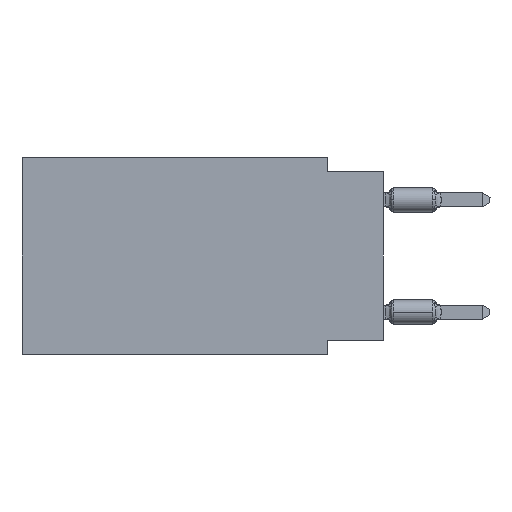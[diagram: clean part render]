
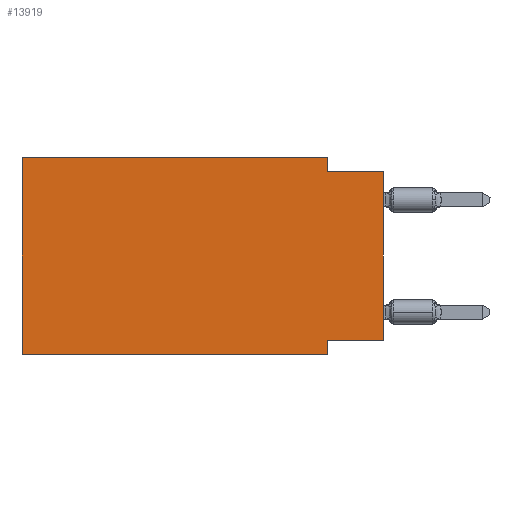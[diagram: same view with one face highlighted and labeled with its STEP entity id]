
A CAD part, left-side view. The second image highlights one B-rep face of the part: STEP entity #13919.
In plain terms, the highlighted planar face has unit normal (-1, 0, 0).
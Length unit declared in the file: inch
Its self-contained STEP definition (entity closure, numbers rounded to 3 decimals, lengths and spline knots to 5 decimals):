
#521 = EDGE_CURVE ( 'NONE', #18550, #58341, #49452, .T. ) ;
#3429 = CARTESIAN_POINT ( 'NONE',  ( 0., 0.1, 0. ) ) ;
#7042 = PLANE ( 'NONE',  #61898 ) ;
#7747 = FACE_OUTER_BOUND ( 'NONE', #23173, .T. ) ;
#7822 = CARTESIAN_POINT ( 'NONE',  ( 0., 0., 0. ) ) ;
#8742 = ORIENTED_EDGE ( 'NONE', *, *, #59085, .F. ) ;
#11381 = CARTESIAN_POINT ( 'NONE',  ( 0., 0.1, -0.025 ) ) ;
#11712 = CARTESIAN_POINT ( 'NONE',  ( 0., 0.1, -0.35 ) ) ;
#11769 = VERTEX_POINT ( 'NONE', #45825 ) ;
#12940 = VECTOR ( 'NONE', #59813, 39.37008 ) ;
#13713 = LINE ( 'NONE', #46192, #62408 ) ;
#13919 = ADVANCED_FACE ( 'NONE', ( #7747 ), #7042, .F. ) ;
#14880 = VERTEX_POINT ( 'NONE', #69265 ) ;
#18035 = LINE ( 'NONE', #50842, #18871 ) ;
#18550 = VERTEX_POINT ( 'NONE', #19063 ) ;
#18871 = VECTOR ( 'NONE', #55851, 39.37008 ) ;
#19063 = CARTESIAN_POINT ( 'NONE',  ( 0., 0.1, -0.325 ) ) ;
#20059 = VECTOR ( 'NONE', #61275, 39.37008 ) ;
#21647 = DIRECTION ( 'NONE',  ( 0., 1., 0. ) ) ;
#23173 = EDGE_LOOP ( 'NONE', ( #65685, #52753, #58268, #8742, #44188, #50461, #50908, #44520 ) ) ;
#24486 = DIRECTION ( 'NONE',  ( 1., 0., 0. ) ) ;
#24844 = DIRECTION ( 'NONE',  ( 0., -1., 0. ) ) ;
#25246 = EDGE_CURVE ( 'NONE', #11769, #18550, #44127, .T. ) ;
#28742 = CARTESIAN_POINT ( 'NONE',  ( 0., 0.1, -0.35 ) ) ;
#28790 = CARTESIAN_POINT ( 'NONE',  ( 0., 0.645, 0. ) ) ;
#29595 = DIRECTION ( 'NONE',  ( 0., 0., 1. ) ) ;
#29667 = CARTESIAN_POINT ( 'NONE',  ( 0., 0.645, 0. ) ) ;
#29849 = DIRECTION ( 'NONE',  ( 0., 0., -1. ) ) ;
#30200 = VECTOR ( 'NONE', #21647, 39.37008 ) ;
#30280 = EDGE_CURVE ( 'NONE', #43369, #59785, #53314, .T. ) ;
#32622 = CARTESIAN_POINT ( 'NONE',  ( 0., 0.1, 0. ) ) ;
#32871 = EDGE_CURVE ( 'NONE', #56341, #39879, #18035, .T. ) ;
#32896 = VECTOR ( 'NONE', #43656, 39.37008 ) ;
#33381 = EDGE_CURVE ( 'NONE', #59785, #14880, #55222, .T. ) ;
#36158 = VECTOR ( 'NONE', #24844, 39.37008 ) ;
#37838 = EDGE_CURVE ( 'NONE', #11769, #14880, #56710, .T. ) ;
#38838 = CARTESIAN_POINT ( 'NONE',  ( 0., 0., -0.025 ) ) ;
#39879 = VERTEX_POINT ( 'NONE', #29667 ) ;
#40134 = DIRECTION ( 'NONE',  ( 0., -1., 0. ) ) ;
#40177 = CARTESIAN_POINT ( 'NONE',  ( 0., 0.645, -0.35 ) ) ;
#43369 = VERTEX_POINT ( 'NONE', #3429 ) ;
#43656 = DIRECTION ( 'NONE',  ( 0., 0., -1. ) ) ;
#44127 = LINE ( 'NONE', #54474, #30200 ) ;
#44188 = ORIENTED_EDGE ( 'NONE', *, *, #32871, .F. ) ;
#44520 = ORIENTED_EDGE ( 'NONE', *, *, #25246, .F. ) ;
#44540 = EDGE_CURVE ( 'NONE', #56341, #58341, #51948, .T. ) ;
#45825 = CARTESIAN_POINT ( 'NONE',  ( 0., 0., -0.325 ) ) ;
#46192 = CARTESIAN_POINT ( 'NONE',  ( 0., 0.645, 0. ) ) ;
#49452 = LINE ( 'NONE', #28742, #12940 ) ;
#50461 = ORIENTED_EDGE ( 'NONE', *, *, #44540, .T. ) ;
#50842 = CARTESIAN_POINT ( 'NONE',  ( 0., 0.645, 0. ) ) ;
#50908 = ORIENTED_EDGE ( 'NONE', *, *, #521, .F. ) ;
#51948 = LINE ( 'NONE', #40177, #36158 ) ;
#52753 = ORIENTED_EDGE ( 'NONE', *, *, #33381, .F. ) ;
#53314 = LINE ( 'NONE', #32622, #32896 ) ;
#54474 = CARTESIAN_POINT ( 'NONE',  ( 0., 0., -0.325 ) ) ;
#55222 = LINE ( 'NONE', #38838, #20059 ) ;
#55851 = DIRECTION ( 'NONE',  ( 0., 0., 1. ) ) ;
#56341 = VERTEX_POINT ( 'NONE', #64556 ) ;
#56710 = LINE ( 'NONE', #7822, #69335 ) ;
#58268 = ORIENTED_EDGE ( 'NONE', *, *, #30280, .F. ) ;
#58341 = VERTEX_POINT ( 'NONE', #11712 ) ;
#59085 = EDGE_CURVE ( 'NONE', #39879, #43369, #13713, .T. ) ;
#59785 = VERTEX_POINT ( 'NONE', #11381 ) ;
#59813 = DIRECTION ( 'NONE',  ( 0., 0., -1. ) ) ;
#61275 = DIRECTION ( 'NONE',  ( 0., -1., 0. ) ) ;
#61898 = AXIS2_PLACEMENT_3D ( 'NONE', #28790, #24486, #29849 ) ;
#62408 = VECTOR ( 'NONE', #40134, 39.37008 ) ;
#64556 = CARTESIAN_POINT ( 'NONE',  ( 0., 0.645, -0.35 ) ) ;
#65685 = ORIENTED_EDGE ( 'NONE', *, *, #37838, .T. ) ;
#69265 = CARTESIAN_POINT ( 'NONE',  ( 0., 0., -0.025 ) ) ;
#69335 = VECTOR ( 'NONE', #29595, 39.37008 ) ;
